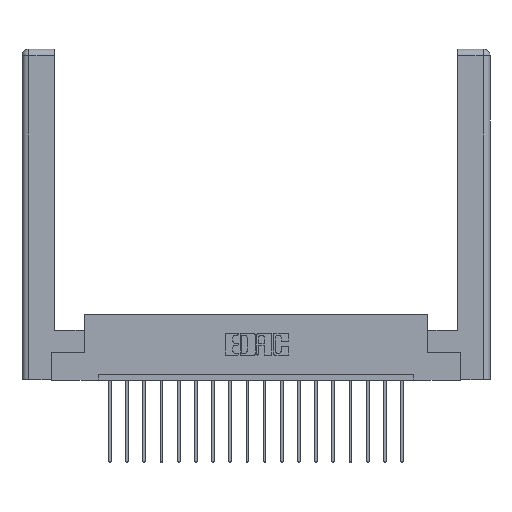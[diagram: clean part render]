
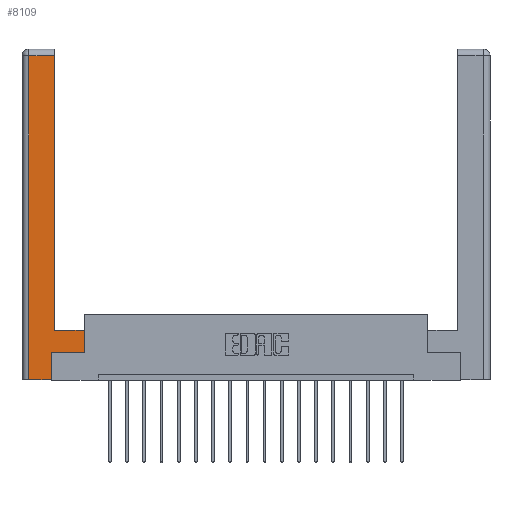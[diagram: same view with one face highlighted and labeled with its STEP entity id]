
A CAD part, top view. The second image highlights one B-rep face of the part: STEP entity #8109.
In plain terms, the highlighted planar face has unit normal (0, 0, 1).
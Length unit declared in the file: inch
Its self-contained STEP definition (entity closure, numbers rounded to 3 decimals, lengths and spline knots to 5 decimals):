
#440 = EDGE_CURVE ( 'NONE', #8246, #3316, #13254, .T. ) ;
#491 = LINE ( 'NONE', #8187, #6736 ) ;
#810 = DIRECTION ( 'NONE',  ( -1., 0., 0. ) ) ;
#975 = CARTESIAN_POINT ( 'NONE',  ( 0.565, 0.45, 0. ) ) ;
#1247 = ORIENTED_EDGE ( 'NONE', *, *, #13625, .T. ) ;
#1897 = CARTESIAN_POINT ( 'NONE',  ( 0.295, 3., 0. ) ) ;
#2086 = CARTESIAN_POINT ( 'NONE',  ( 0.265, 0., 0. ) ) ;
#2250 = EDGE_CURVE ( 'NONE', #14317, #11933, #10187, .T. ) ;
#2288 = DIRECTION ( 'NONE',  ( 1., 0., 0. ) ) ;
#2368 = EDGE_CURVE ( 'NONE', #2791, #14524, #8281, .T. ) ;
#2432 = FACE_OUTER_BOUND ( 'NONE', #2902, .T. ) ;
#2791 = VERTEX_POINT ( 'NONE', #11144 ) ;
#2902 = EDGE_LOOP ( 'NONE', ( #17296, #18151, #17923, #14576, #5772, #15631, #1247, #17592 ) ) ;
#2941 = CARTESIAN_POINT ( 'NONE',  ( 0.295, 0.45, 0. ) ) ;
#3189 = VECTOR ( 'NONE', #2288, 39.37008 ) ;
#3316 = VERTEX_POINT ( 'NONE', #2941 ) ;
#3805 = CARTESIAN_POINT ( 'NONE',  ( 0.295, 2.94, 0. ) ) ;
#4511 = EDGE_CURVE ( 'NONE', #14045, #7732, #491, .T. ) ;
#5192 = DIRECTION ( 'NONE',  ( 0., 0., -1. ) ) ;
#5320 = VECTOR ( 'NONE', #13820, 39.37008 ) ;
#5738 = LINE ( 'NONE', #7487, #17553 ) ;
#5772 = ORIENTED_EDGE ( 'NONE', *, *, #15521, .T. ) ;
#5892 = VECTOR ( 'NONE', #17896, 39.37008 ) ;
#6248 = EDGE_CURVE ( 'NONE', #7732, #2791, #5738, .T. ) ;
#6300 = VECTOR ( 'NONE', #810, 39.37008 ) ;
#6435 = DIRECTION ( 'NONE',  ( 0., 1., 0. ) ) ;
#6483 = CARTESIAN_POINT ( 'NONE',  ( 0.565, 0.245, 0. ) ) ;
#6592 = DIRECTION ( 'NONE',  ( -1., 0., 0. ) ) ;
#6736 = VECTOR ( 'NONE', #8248, 39.37008 ) ;
#6949 = VECTOR ( 'NONE', #6435, 39.37008 ) ;
#7487 = CARTESIAN_POINT ( 'NONE',  ( 0.0615, 0., 0. ) ) ;
#7732 = VERTEX_POINT ( 'NONE', #18882 ) ;
#8109 = ADVANCED_FACE ( 'NONE', ( #2432 ), #15062, .F. ) ;
#8187 = CARTESIAN_POINT ( 'NONE',  ( 0.0615, 2.94, 0. ) ) ;
#8246 = VERTEX_POINT ( 'NONE', #975 ) ;
#8248 = DIRECTION ( 'NONE',  ( -1., 0., 0. ) ) ;
#8281 = LINE ( 'NONE', #2086, #3189 ) ;
#8819 = EDGE_CURVE ( 'NONE', #3316, #14045, #16515, .T. ) ;
#9368 = CARTESIAN_POINT ( 'NONE',  ( 0.265, 0.245, 0. ) ) ;
#10187 = LINE ( 'NONE', #10726, #12220 ) ;
#10726 = CARTESIAN_POINT ( 'NONE',  ( 0.565, 0.245, 0. ) ) ;
#11144 = CARTESIAN_POINT ( 'NONE',  ( 0.0615, 0., 0. ) ) ;
#11933 = VERTEX_POINT ( 'NONE', #6483 ) ;
#12220 = VECTOR ( 'NONE', #16614, 39.37008 ) ;
#13254 = LINE ( 'NONE', #18532, #6300 ) ;
#13625 = EDGE_CURVE ( 'NONE', #11933, #8246, #17108, .T. ) ;
#13820 = DIRECTION ( 'NONE',  ( 0., 1., 0. ) ) ;
#14045 = VERTEX_POINT ( 'NONE', #3805 ) ;
#14317 = VERTEX_POINT ( 'NONE', #17201 ) ;
#14524 = VERTEX_POINT ( 'NONE', #17152 ) ;
#14576 = ORIENTED_EDGE ( 'NONE', *, *, #2368, .T. ) ;
#15062 = PLANE ( 'NONE',  #17946 ) ;
#15216 = CARTESIAN_POINT ( 'NONE',  ( 0.565, 0.45, 0. ) ) ;
#15521 = EDGE_CURVE ( 'NONE', #14524, #14317, #16190, .T. ) ;
#15631 = ORIENTED_EDGE ( 'NONE', *, *, #2250, .T. ) ;
#16190 = LINE ( 'NONE', #9368, #6949 ) ;
#16480 = CARTESIAN_POINT ( 'NONE',  ( 0., 0., 0. ) ) ;
#16515 = LINE ( 'NONE', #1897, #5892 ) ;
#16614 = DIRECTION ( 'NONE',  ( 1., 0., 0. ) ) ;
#17108 = LINE ( 'NONE', #15216, #5320 ) ;
#17152 = CARTESIAN_POINT ( 'NONE',  ( 0.265, 0., 0. ) ) ;
#17201 = CARTESIAN_POINT ( 'NONE',  ( 0.265, 0.245, 0. ) ) ;
#17296 = ORIENTED_EDGE ( 'NONE', *, *, #8819, .T. ) ;
#17553 = VECTOR ( 'NONE', #17846, 39.37008 ) ;
#17592 = ORIENTED_EDGE ( 'NONE', *, *, #440, .T. ) ;
#17846 = DIRECTION ( 'NONE',  ( 0., -1., 0. ) ) ;
#17896 = DIRECTION ( 'NONE',  ( 0., 1., 0. ) ) ;
#17923 = ORIENTED_EDGE ( 'NONE', *, *, #6248, .T. ) ;
#17946 = AXIS2_PLACEMENT_3D ( 'NONE', #16480, #5192, #6592 ) ;
#18151 = ORIENTED_EDGE ( 'NONE', *, *, #4511, .T. ) ;
#18532 = CARTESIAN_POINT ( 'NONE',  ( 0.295, 0.45, 0. ) ) ;
#18882 = CARTESIAN_POINT ( 'NONE',  ( 0.0615, 2.94, 0. ) ) ;
